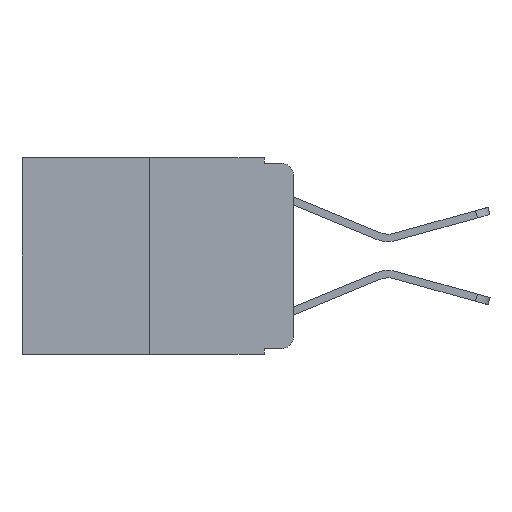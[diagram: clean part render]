
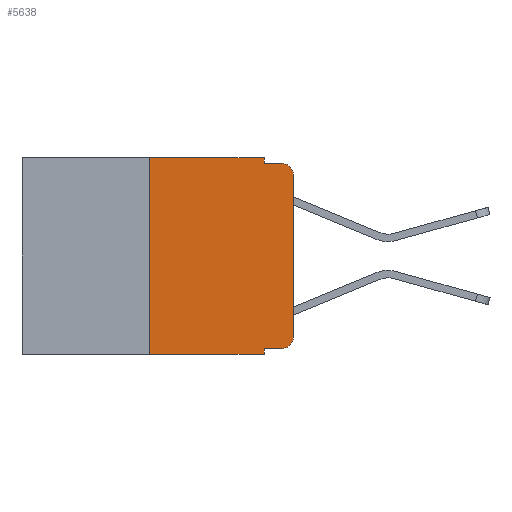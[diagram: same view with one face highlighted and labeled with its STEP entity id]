
A CAD part, left-side view. The second image highlights one B-rep face of the part: STEP entity #5638.
In plain terms, the highlighted planar face has unit normal (-1, 0, 0).
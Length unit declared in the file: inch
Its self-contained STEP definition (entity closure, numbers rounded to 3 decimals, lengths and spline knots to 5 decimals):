
#32 = VERTEX_POINT ( 'NONE', #15364 ) ;
#321 = VECTOR ( 'NONE', #13292, 39.37008 ) ;
#423 = CARTESIAN_POINT ( 'NONE',  ( 0., 0.051, -0.01 ) ) ;
#621 = AXIS2_PLACEMENT_3D ( 'NONE', #1077, #12608, #1021 ) ;
#833 = CARTESIAN_POINT ( 'NONE',  ( 0., 0., -0.03 ) ) ;
#898 = ORIENTED_EDGE ( 'NONE', *, *, #11238, .T. ) ;
#1021 = DIRECTION ( 'NONE',  ( 0., 0., -1. ) ) ;
#1077 = CARTESIAN_POINT ( 'NONE',  ( 0., 0.473, 0. ) ) ;
#1313 = CIRCLE ( 'NONE', #2909, 0.02 ) ;
#1774 = CIRCLE ( 'NONE', #4494, 0.02 ) ;
#1780 = EDGE_CURVE ( 'NONE', #8602, #16073, #6847, .T. ) ;
#2909 = AXIS2_PLACEMENT_3D ( 'NONE', #12373, #7900, #16524 ) ;
#3103 = DIRECTION ( 'NONE',  ( 0., -1., 0. ) ) ;
#3116 = LINE ( 'NONE', #3956, #18058 ) ;
#3353 = VECTOR ( 'NONE', #14854, 39.37008 ) ;
#3777 = LINE ( 'NONE', #4532, #15971 ) ;
#3888 = CARTESIAN_POINT ( 'NONE',  ( 0., 0.25, 0. ) ) ;
#3909 = CARTESIAN_POINT ( 'NONE',  ( 0., 0.051, -0.01 ) ) ;
#3956 = CARTESIAN_POINT ( 'NONE',  ( 0., 0., 0. ) ) ;
#3957 = EDGE_CURVE ( 'NONE', #13886, #16309, #12427, .T. ) ;
#4075 = CARTESIAN_POINT ( 'NONE',  ( 0., 0.051, 0. ) ) ;
#4084 = ORIENTED_EDGE ( 'NONE', *, *, #5487, .T. ) ;
#4277 = DIRECTION ( 'NONE',  ( 0., 0., -1. ) ) ;
#4474 = ORIENTED_EDGE ( 'NONE', *, *, #3957, .T. ) ;
#4494 = AXIS2_PLACEMENT_3D ( 'NONE', #12001, #13508, #9261 ) ;
#4532 = CARTESIAN_POINT ( 'NONE',  ( 0., 0.051, 0. ) ) ;
#4861 = EDGE_LOOP ( 'NONE', ( #7697, #4084, #11988, #14912, #16598, #15018, #898, #8367, #4474, #8843 ) ) ;
#5162 = VECTOR ( 'NONE', #9655, 39.37008 ) ;
#5333 = EDGE_CURVE ( 'NONE', #16309, #5379, #1774, .T. ) ;
#5379 = VERTEX_POINT ( 'NONE', #6389 ) ;
#5412 = VERTEX_POINT ( 'NONE', #16401 ) ;
#5487 = EDGE_CURVE ( 'NONE', #12040, #5976, #1313, .T. ) ;
#5638 = ADVANCED_FACE ( 'NONE', ( #14862 ), #6815, .F. ) ;
#5976 = VERTEX_POINT ( 'NONE', #6257 ) ;
#6257 = CARTESIAN_POINT ( 'NONE',  ( 0., 0.02, -0.01 ) ) ;
#6389 = CARTESIAN_POINT ( 'NONE',  ( 0., 0., -0.313 ) ) ;
#6474 = EDGE_CURVE ( 'NONE', #10100, #5976, #6590, .T. ) ;
#6590 = LINE ( 'NONE', #423, #15334 ) ;
#6815 = PLANE ( 'NONE',  #621 ) ;
#6847 = LINE ( 'NONE', #11846, #321 ) ;
#7697 = ORIENTED_EDGE ( 'NONE', *, *, #12798, .T. ) ;
#7900 = DIRECTION ( 'NONE',  ( -1., 0., 0. ) ) ;
#8367 = ORIENTED_EDGE ( 'NONE', *, *, #14533, .F. ) ;
#8548 = LINE ( 'NONE', #17602, #13713 ) ;
#8602 = VERTEX_POINT ( 'NONE', #18259 ) ;
#8843 = ORIENTED_EDGE ( 'NONE', *, *, #5333, .T. ) ;
#9080 = CARTESIAN_POINT ( 'NONE',  ( 0., 0.051, 0. ) ) ;
#9142 = CARTESIAN_POINT ( 'NONE',  ( 0., 0.02, -0.333 ) ) ;
#9261 = DIRECTION ( 'NONE',  ( 0., 0., -1. ) ) ;
#9655 = DIRECTION ( 'NONE',  ( 0., 0., 1. ) ) ;
#10100 = VERTEX_POINT ( 'NONE', #3909 ) ;
#10307 = CARTESIAN_POINT ( 'NONE',  ( 0., 0.051, -0.333 ) ) ;
#10644 = EDGE_CURVE ( 'NONE', #32, #8602, #13726, .T. ) ;
#11238 = EDGE_CURVE ( 'NONE', #32, #5412, #8548, .T. ) ;
#11720 = DIRECTION ( 'NONE',  ( 0., -1., 0. ) ) ;
#11846 = CARTESIAN_POINT ( 'NONE',  ( 0., 0.473, 0. ) ) ;
#11988 = ORIENTED_EDGE ( 'NONE', *, *, #6474, .F. ) ;
#12001 = CARTESIAN_POINT ( 'NONE',  ( 0., 0.02, -0.313 ) ) ;
#12040 = VERTEX_POINT ( 'NONE', #833 ) ;
#12373 = CARTESIAN_POINT ( 'NONE',  ( 0., 0.02, -0.03 ) ) ;
#12427 = LINE ( 'NONE', #10307, #14222 ) ;
#12595 = LINE ( 'NONE', #9080, #3353 ) ;
#12608 = DIRECTION ( 'NONE',  ( 1., 0., 0. ) ) ;
#12798 = EDGE_CURVE ( 'NONE', #5379, #12040, #3116, .T. ) ;
#13292 = DIRECTION ( 'NONE',  ( 0., -1., 0. ) ) ;
#13508 = DIRECTION ( 'NONE',  ( -1., 0., 0. ) ) ;
#13688 = CARTESIAN_POINT ( 'NONE',  ( 0., 0.051, -0.333 ) ) ;
#13713 = VECTOR ( 'NONE', #14732, 39.37008 ) ;
#13726 = LINE ( 'NONE', #3888, #5162 ) ;
#13886 = VERTEX_POINT ( 'NONE', #13688 ) ;
#14222 = VECTOR ( 'NONE', #3103, 39.37008 ) ;
#14533 = EDGE_CURVE ( 'NONE', #13886, #5412, #12595, .T. ) ;
#14732 = DIRECTION ( 'NONE',  ( 0., -1., 0. ) ) ;
#14854 = DIRECTION ( 'NONE',  ( 0., 0., -1. ) ) ;
#14862 = FACE_OUTER_BOUND ( 'NONE', #4861, .T. ) ;
#14912 = ORIENTED_EDGE ( 'NONE', *, *, #15667, .F. ) ;
#15018 = ORIENTED_EDGE ( 'NONE', *, *, #10644, .F. ) ;
#15334 = VECTOR ( 'NONE', #11720, 39.37008 ) ;
#15364 = CARTESIAN_POINT ( 'NONE',  ( 0., 0.25, -0.343 ) ) ;
#15667 = EDGE_CURVE ( 'NONE', #16073, #10100, #3777, .T. ) ;
#15971 = VECTOR ( 'NONE', #4277, 39.37008 ) ;
#16073 = VERTEX_POINT ( 'NONE', #4075 ) ;
#16309 = VERTEX_POINT ( 'NONE', #9142 ) ;
#16401 = CARTESIAN_POINT ( 'NONE',  ( 0., 0.051, -0.343 ) ) ;
#16524 = DIRECTION ( 'NONE',  ( 0., 0., -1. ) ) ;
#16598 = ORIENTED_EDGE ( 'NONE', *, *, #1780, .F. ) ;
#17602 = CARTESIAN_POINT ( 'NONE',  ( 0., 0.473, -0.343 ) ) ;
#18058 = VECTOR ( 'NONE', #18510, 39.37008 ) ;
#18259 = CARTESIAN_POINT ( 'NONE',  ( 0., 0.25, 0. ) ) ;
#18510 = DIRECTION ( 'NONE',  ( 0., 0., 1. ) ) ;
